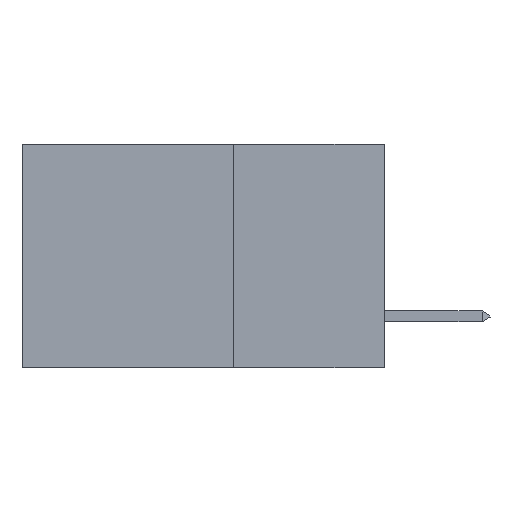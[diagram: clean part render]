
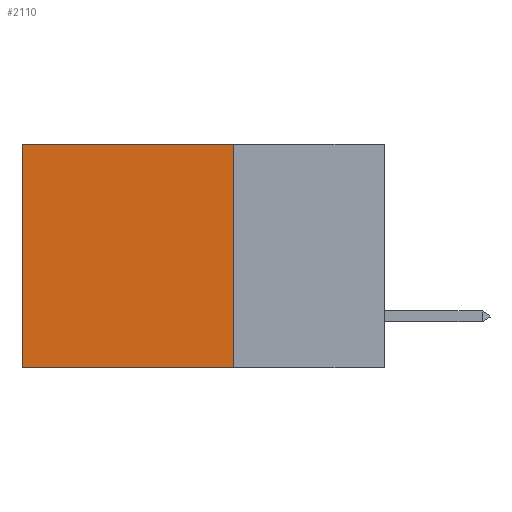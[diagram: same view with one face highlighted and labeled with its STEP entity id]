
A CAD part, left-side view. The second image highlights one B-rep face of the part: STEP entity #2110.
In plain terms, the highlighted planar face has unit normal (-1, 0, 0).
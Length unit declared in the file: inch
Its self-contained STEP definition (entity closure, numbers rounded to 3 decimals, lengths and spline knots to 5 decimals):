
#1578 = EDGE_CURVE ( 'NONE', #27111, #15789, #11241, .T. ) ;
#2110 = ADVANCED_FACE ( 'NONE', ( #26478 ), #3862, .F. ) ;
#2592 = VERTEX_POINT ( 'NONE', #19365 ) ;
#3647 = LINE ( 'NONE', #15961, #16786 ) ;
#3862 = PLANE ( 'NONE',  #21427 ) ;
#5944 = LINE ( 'NONE', #10369, #14369 ) ;
#8113 = CARTESIAN_POINT ( 'NONE',  ( 0.2875, 0.25, 0. ) ) ;
#10033 = EDGE_CURVE ( 'NONE', #2592, #27468, #17246, .T. ) ;
#10369 = CARTESIAN_POINT ( 'NONE',  ( 0.2875, 0.25, 0. ) ) ;
#11241 = LINE ( 'NONE', #25639, #21381 ) ;
#11860 = EDGE_CURVE ( 'NONE', #15789, #27468, #3647, .T. ) ;
#13662 = DIRECTION ( 'NONE',  ( 0., 1., 0. ) ) ;
#14369 = VECTOR ( 'NONE', #20199, 39.37008 ) ;
#14489 = ORIENTED_EDGE ( 'NONE', *, *, #11860, .T. ) ;
#14888 = DIRECTION ( 'NONE',  ( 1., 0., 0. ) ) ;
#15419 = EDGE_CURVE ( 'NONE', #27111, #2592, #5944, .T. ) ;
#15623 = CARTESIAN_POINT ( 'NONE',  ( 0.2875, 0.25, -0.37 ) ) ;
#15789 = VERTEX_POINT ( 'NONE', #27040 ) ;
#15961 = CARTESIAN_POINT ( 'NONE',  ( 0.2875, 0.6, 0. ) ) ;
#16786 = VECTOR ( 'NONE', #22588, 39.37008 ) ;
#17038 = DIRECTION ( 'NONE',  ( 0., 0., -1. ) ) ;
#17246 = LINE ( 'NONE', #15623, #21987 ) ;
#18641 = ORIENTED_EDGE ( 'NONE', *, *, #1578, .T. ) ;
#19187 = ORIENTED_EDGE ( 'NONE', *, *, #10033, .F. ) ;
#19365 = CARTESIAN_POINT ( 'NONE',  ( 0.2875, 0.25, -0.37 ) ) ;
#20199 = DIRECTION ( 'NONE',  ( 0., 0., -1. ) ) ;
#21192 = DIRECTION ( 'NONE',  ( 0., 1., 0. ) ) ;
#21381 = VECTOR ( 'NONE', #21192, 39.37008 ) ;
#21427 = AXIS2_PLACEMENT_3D ( 'NONE', #8113, #14888, #17038 ) ;
#21987 = VECTOR ( 'NONE', #13662, 39.37008 ) ;
#22318 = ORIENTED_EDGE ( 'NONE', *, *, #15419, .F. ) ;
#22588 = DIRECTION ( 'NONE',  ( 0., 0., -1. ) ) ;
#24014 = CARTESIAN_POINT ( 'NONE',  ( 0.2875, 0.25, 0. ) ) ;
#24644 = EDGE_LOOP ( 'NONE', ( #14489, #19187, #22318, #18641 ) ) ;
#25639 = CARTESIAN_POINT ( 'NONE',  ( 0.2875, 0.25, 0. ) ) ;
#26134 = CARTESIAN_POINT ( 'NONE',  ( 0.2875, 0.6, -0.37 ) ) ;
#26478 = FACE_OUTER_BOUND ( 'NONE', #24644, .T. ) ;
#27040 = CARTESIAN_POINT ( 'NONE',  ( 0.2875, 0.6, 0. ) ) ;
#27111 = VERTEX_POINT ( 'NONE', #24014 ) ;
#27468 = VERTEX_POINT ( 'NONE', #26134 ) ;
